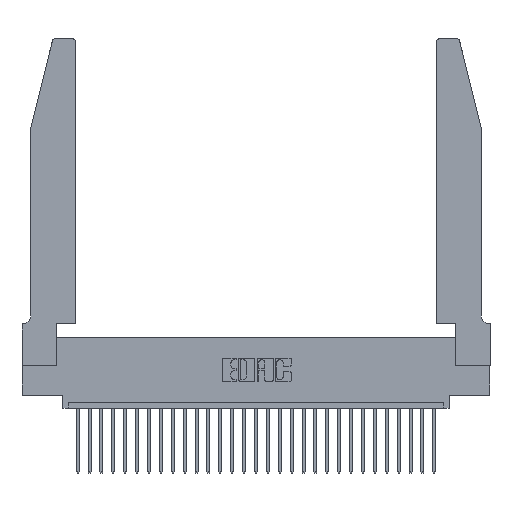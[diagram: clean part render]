
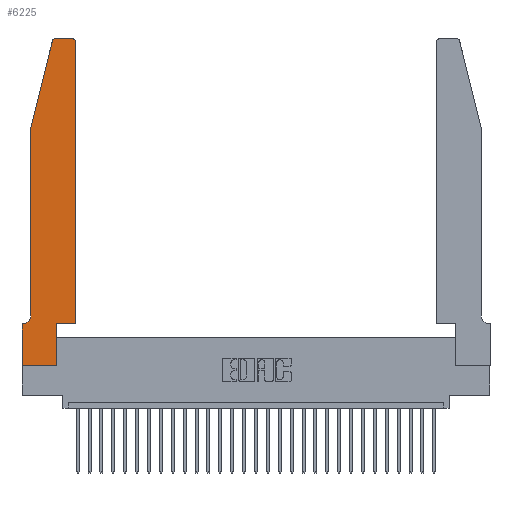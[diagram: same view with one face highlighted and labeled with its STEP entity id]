
A CAD part, top view. The second image highlights one B-rep face of the part: STEP entity #6225.
In plain terms, the highlighted planar face has unit normal (0, 0, 1).
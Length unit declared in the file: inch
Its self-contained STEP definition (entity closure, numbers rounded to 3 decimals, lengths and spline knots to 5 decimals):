
#204 = CARTESIAN_POINT ( 'NONE',  ( 0.25487, 2.72718, 0.37 ) ) ;
#391 = VERTEX_POINT ( 'NONE', #19121 ) ;
#421 = EDGE_LOOP ( 'NONE', ( #2128, #6961, #25918, #22899, #6259, #15807, #10744, #19621, #22202, #3876, #5862, #29147 ) ) ;
#1223 = LINE ( 'NONE', #3231, #29578 ) ;
#1280 = CARTESIAN_POINT ( 'NONE',  ( 0.0755, 2., 0.37 ) ) ;
#2128 = ORIENTED_EDGE ( 'NONE', *, *, #23838, .T. ) ;
#3098 = EDGE_CURVE ( 'NONE', #25629, #22246, #4081, .T. ) ;
#3231 = CARTESIAN_POINT ( 'NONE',  ( 0., 0., 0.37 ) ) ;
#3599 = LINE ( 'NONE', #19591, #11552 ) ;
#3876 = ORIENTED_EDGE ( 'NONE', *, *, #19044, .T. ) ;
#4081 = CIRCLE ( 'NONE', #7720, 0.03 ) ;
#4235 = CARTESIAN_POINT ( 'NONE',  ( 0.2605, 2.75, 0.37 ) ) ;
#4245 = DIRECTION ( 'NONE',  ( 0., 0., 1. ) ) ;
#4626 = VECTOR ( 'NONE', #8568, 39.37008 ) ;
#4817 = CIRCLE ( 'NONE', #20941, 0.03 ) ;
#4949 = DIRECTION ( 'NONE',  ( 1., 0., 0. ) ) ;
#5288 = CARTESIAN_POINT ( 'NONE',  ( 0.2865, 0.35, 0.37 ) ) ;
#5343 = DIRECTION ( 'NONE',  ( 0., -1., 0. ) ) ;
#5431 = CARTESIAN_POINT ( 'NONE',  ( 0.0055, 0.35, 0.37 ) ) ;
#5458 = CARTESIAN_POINT ( 'NONE',  ( 0., 0., 0.37 ) ) ;
#5537 = CARTESIAN_POINT ( 'NONE',  ( 0.4505, 0.35, 0.37 ) ) ;
#5543 = CARTESIAN_POINT ( 'NONE',  ( 0., 0.35, 0.37 ) ) ;
#5554 = EDGE_CURVE ( 'NONE', #16924, #20329, #3599, .T. ) ;
#5581 = LINE ( 'NONE', #5458, #11376 ) ;
#5698 = AXIS2_PLACEMENT_3D ( 'NONE', #18158, #15758, #29207 ) ;
#5771 = CIRCLE ( 'NONE', #5698, 0.07 ) ;
#5862 = ORIENTED_EDGE ( 'NONE', *, *, #27176, .T. ) ;
#5944 = DIRECTION ( 'NONE',  ( 1., 0., 0. ) ) ;
#6225 = ADVANCED_FACE ( 'NONE', ( #13643 ), #13892, .T. ) ;
#6259 = ORIENTED_EDGE ( 'NONE', *, *, #22177, .T. ) ;
#6961 = ORIENTED_EDGE ( 'NONE', *, *, #26065, .T. ) ;
#7682 = DIRECTION ( 'NONE',  ( 1., 0., 0. ) ) ;
#7720 = AXIS2_PLACEMENT_3D ( 'NONE', #15110, #26784, #8196 ) ;
#8196 = DIRECTION ( 'NONE',  ( 1., 0., 0. ) ) ;
#8568 = DIRECTION ( 'NONE',  ( -1., 0., 0. ) ) ;
#9191 = VERTEX_POINT ( 'NONE', #5431 ) ;
#9456 = DIRECTION ( 'NONE',  ( 0., 0., 1. ) ) ;
#9955 = CARTESIAN_POINT ( 'NONE',  ( 0.0755, 0.35, 0.37 ) ) ;
#9998 = VERTEX_POINT ( 'NONE', #23565 ) ;
#10503 = EDGE_CURVE ( 'NONE', #17977, #19327, #12059, .T. ) ;
#10744 = ORIENTED_EDGE ( 'NONE', *, *, #26153, .T. ) ;
#11376 = VECTOR ( 'NONE', #7682, 39.37008 ) ;
#11440 = CARTESIAN_POINT ( 'NONE',  ( 0.0755, 2., 0.37 ) ) ;
#11552 = VECTOR ( 'NONE', #17905, 39.37008 ) ;
#11664 = LINE ( 'NONE', #9955, #23479 ) ;
#12059 = LINE ( 'NONE', #19800, #16704 ) ;
#12853 = LINE ( 'NONE', #1280, #17512 ) ;
#12879 = LINE ( 'NONE', #15165, #20750 ) ;
#13643 = FACE_OUTER_BOUND ( 'NONE', #421, .T. ) ;
#13892 = PLANE ( 'NONE',  #16851 ) ;
#14283 = EDGE_CURVE ( 'NONE', #26795, #16924, #12853, .T. ) ;
#14710 = CARTESIAN_POINT ( 'NONE',  ( 0.4505, 2.72, 0.37 ) ) ;
#15110 = CARTESIAN_POINT ( 'NONE',  ( 0.4205, 2.72, 0.37 ) ) ;
#15165 = CARTESIAN_POINT ( 'NONE',  ( 0.4505, 0.35, 0.37 ) ) ;
#15432 = CARTESIAN_POINT ( 'NONE',  ( 0.4505, 0.35, 0.37 ) ) ;
#15543 = DIRECTION ( 'NONE',  ( 1., 0., 0. ) ) ;
#15758 = DIRECTION ( 'NONE',  ( 0., 0., -1. ) ) ;
#15807 = ORIENTED_EDGE ( 'NONE', *, *, #26218, .T. ) ;
#16275 = CARTESIAN_POINT ( 'NONE',  ( 0.284, 2.72, 0.37 ) ) ;
#16704 = VECTOR ( 'NONE', #22137, 39.37008 ) ;
#16851 = AXIS2_PLACEMENT_3D ( 'NONE', #5543, #4245, #15543 ) ;
#16924 = VERTEX_POINT ( 'NONE', #11440 ) ;
#17157 = LINE ( 'NONE', #4235, #4626 ) ;
#17512 = VECTOR ( 'NONE', #21937, 39.37008 ) ;
#17528 = EDGE_CURVE ( 'NONE', #9998, #17977, #5581, .T. ) ;
#17905 = DIRECTION ( 'NONE',  ( 0., -1., 0. ) ) ;
#17977 = VERTEX_POINT ( 'NONE', #29742 ) ;
#18158 = CARTESIAN_POINT ( 'NONE',  ( 0.0055, 0.42, 0.37 ) ) ;
#19044 = EDGE_CURVE ( 'NONE', #19327, #23554, #12879, .T. ) ;
#19121 = CARTESIAN_POINT ( 'NONE',  ( 0.284, 2.75, 0.37 ) ) ;
#19327 = VERTEX_POINT ( 'NONE', #5288 ) ;
#19441 = CARTESIAN_POINT ( 'NONE',  ( 0.0755, 0.42, 0.37 ) ) ;
#19591 = CARTESIAN_POINT ( 'NONE',  ( 0.0755, 2., 0.37 ) ) ;
#19621 = ORIENTED_EDGE ( 'NONE', *, *, #17528, .T. ) ;
#19800 = CARTESIAN_POINT ( 'NONE',  ( 0.2865, 0.35, 0.37 ) ) ;
#20329 = VERTEX_POINT ( 'NONE', #19441 ) ;
#20750 = VECTOR ( 'NONE', #5944, 39.37008 ) ;
#20891 = CARTESIAN_POINT ( 'NONE',  ( 0., 0.35, 0.37 ) ) ;
#20941 = AXIS2_PLACEMENT_3D ( 'NONE', #16275, #9456, #4949 ) ;
#21937 = DIRECTION ( 'NONE',  ( -0.239, -0.971, 0. ) ) ;
#22137 = DIRECTION ( 'NONE',  ( 0., 1., 0. ) ) ;
#22177 = EDGE_CURVE ( 'NONE', #20329, #9191, #5771, .T. ) ;
#22202 = ORIENTED_EDGE ( 'NONE', *, *, #10503, .T. ) ;
#22246 = VERTEX_POINT ( 'NONE', #23080 ) ;
#22899 = ORIENTED_EDGE ( 'NONE', *, *, #5554, .T. ) ;
#23050 = LINE ( 'NONE', #15432, #23798 ) ;
#23080 = CARTESIAN_POINT ( 'NONE',  ( 0.4205, 2.75, 0.37 ) ) ;
#23479 = VECTOR ( 'NONE', #23841, 39.37008 ) ;
#23554 = VERTEX_POINT ( 'NONE', #5537 ) ;
#23565 = CARTESIAN_POINT ( 'NONE',  ( 0., 0., 0.37 ) ) ;
#23798 = VECTOR ( 'NONE', #24906, 39.37008 ) ;
#23838 = EDGE_CURVE ( 'NONE', #22246, #391, #17157, .T. ) ;
#23841 = DIRECTION ( 'NONE',  ( -1., 0., 0. ) ) ;
#24597 = VERTEX_POINT ( 'NONE', #20891 ) ;
#24906 = DIRECTION ( 'NONE',  ( 0., 1., 0. ) ) ;
#25629 = VERTEX_POINT ( 'NONE', #14710 ) ;
#25918 = ORIENTED_EDGE ( 'NONE', *, *, #14283, .T. ) ;
#26065 = EDGE_CURVE ( 'NONE', #391, #26795, #4817, .T. ) ;
#26153 = EDGE_CURVE ( 'NONE', #24597, #9998, #1223, .T. ) ;
#26218 = EDGE_CURVE ( 'NONE', #9191, #24597, #11664, .T. ) ;
#26784 = DIRECTION ( 'NONE',  ( 0., 0., 1. ) ) ;
#26795 = VERTEX_POINT ( 'NONE', #204 ) ;
#27176 = EDGE_CURVE ( 'NONE', #23554, #25629, #23050, .T. ) ;
#29147 = ORIENTED_EDGE ( 'NONE', *, *, #3098, .T. ) ;
#29207 = DIRECTION ( 'NONE',  ( -1., 0., 0. ) ) ;
#29578 = VECTOR ( 'NONE', #5343, 39.37008 ) ;
#29742 = CARTESIAN_POINT ( 'NONE',  ( 0.2865, 0., 0.37 ) ) ;
